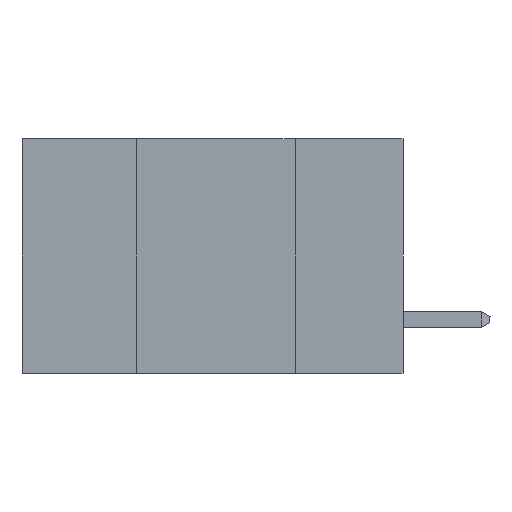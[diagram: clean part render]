
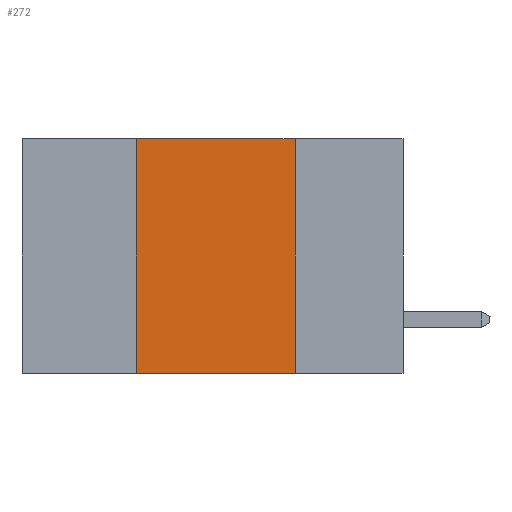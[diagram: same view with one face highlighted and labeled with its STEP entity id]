
A CAD part, left-side view. The second image highlights one B-rep face of the part: STEP entity #272.
In plain terms, the highlighted planar face has unit normal (-1, 0, 0).
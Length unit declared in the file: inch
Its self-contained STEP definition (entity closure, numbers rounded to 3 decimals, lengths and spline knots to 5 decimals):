
#47 = VECTOR ( 'NONE', #8686, 39.37008 ) ;
#54 = ORIENTED_EDGE ( 'NONE', *, *, #7455, .T. ) ;
#272 = ADVANCED_FACE ( 'NONE', ( #20404 ), #5968, .F. ) ;
#307 = EDGE_LOOP ( 'NONE', ( #13438, #16290, #10589, #54 ) ) ;
#1216 = DIRECTION ( 'NONE',  ( 0., 0., -1. ) ) ;
#1860 = EDGE_CURVE ( 'NONE', #18041, #16078, #25192, .T. ) ;
#1935 = VECTOR ( 'NONE', #20901, 39.37008 ) ;
#2629 = CARTESIAN_POINT ( 'NONE',  ( 0., 0.42, 0. ) ) ;
#3502 = CARTESIAN_POINT ( 'NONE',  ( 0., 0.6, 0. ) ) ;
#3845 = CARTESIAN_POINT ( 'NONE',  ( 0., 0.17, -0.37 ) ) ;
#4542 = VERTEX_POINT ( 'NONE', #8023 ) ;
#4787 = DIRECTION ( 'NONE',  ( 0., 0., 1. ) ) ;
#5968 = PLANE ( 'NONE',  #18571 ) ;
#7455 = EDGE_CURVE ( 'NONE', #4542, #16078, #8221, .T. ) ;
#8023 = CARTESIAN_POINT ( 'NONE',  ( 0., 0.42, -0.37 ) ) ;
#8134 = EDGE_CURVE ( 'NONE', #4542, #21067, #9302, .T. ) ;
#8221 = LINE ( 'NONE', #14998, #47 ) ;
#8686 = DIRECTION ( 'NONE',  ( 0., -1., 0. ) ) ;
#8910 = LINE ( 'NONE', #15929, #19924 ) ;
#9302 = LINE ( 'NONE', #2629, #21079 ) ;
#10589 = ORIENTED_EDGE ( 'NONE', *, *, #8134, .F. ) ;
#10849 = CARTESIAN_POINT ( 'NONE',  ( 0., 0.17, 0. ) ) ;
#12305 = EDGE_CURVE ( 'NONE', #21067, #18041, #8910, .T. ) ;
#13438 = ORIENTED_EDGE ( 'NONE', *, *, #1860, .F. ) ;
#14998 = CARTESIAN_POINT ( 'NONE',  ( 0., 0.6, -0.37 ) ) ;
#15643 = CARTESIAN_POINT ( 'NONE',  ( 0., 0.42, 0. ) ) ;
#15929 = CARTESIAN_POINT ( 'NONE',  ( 0., 0.6, 0. ) ) ;
#16078 = VERTEX_POINT ( 'NONE', #3845 ) ;
#16123 = DIRECTION ( 'NONE',  ( 0., -1., 0. ) ) ;
#16290 = ORIENTED_EDGE ( 'NONE', *, *, #12305, .F. ) ;
#18041 = VERTEX_POINT ( 'NONE', #10849 ) ;
#18571 = AXIS2_PLACEMENT_3D ( 'NONE', #3502, #24932, #1216 ) ;
#19924 = VECTOR ( 'NONE', #16123, 39.37008 ) ;
#20404 = FACE_OUTER_BOUND ( 'NONE', #307, .T. ) ;
#20901 = DIRECTION ( 'NONE',  ( 0., 0., -1. ) ) ;
#21067 = VERTEX_POINT ( 'NONE', #15643 ) ;
#21079 = VECTOR ( 'NONE', #4787, 39.37008 ) ;
#24932 = DIRECTION ( 'NONE',  ( 1., 0., 0. ) ) ;
#25192 = LINE ( 'NONE', #30203, #1935 ) ;
#30203 = CARTESIAN_POINT ( 'NONE',  ( 0., 0.17, 0. ) ) ;
